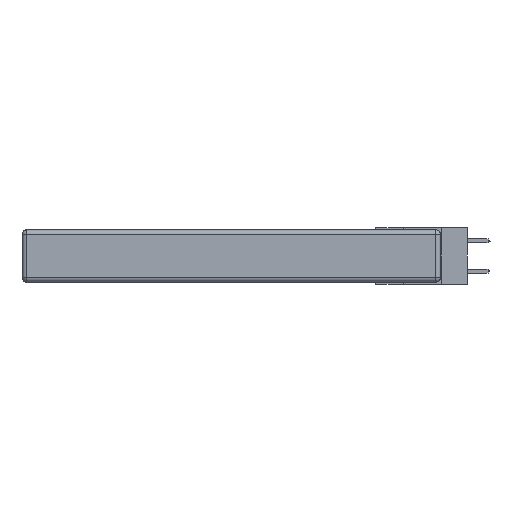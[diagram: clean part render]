
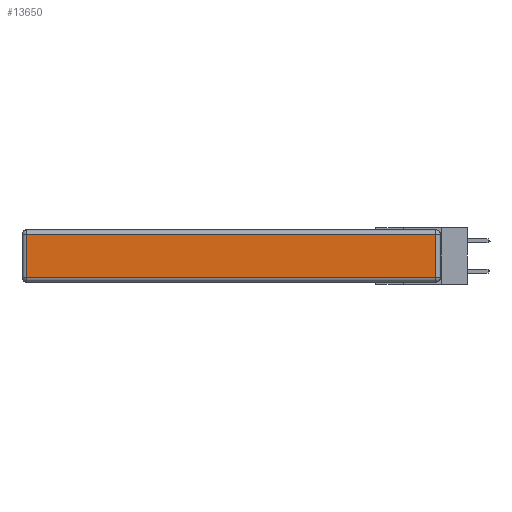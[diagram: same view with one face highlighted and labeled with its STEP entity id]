
A CAD part, left-side view. The second image highlights one B-rep face of the part: STEP entity #13650.
In plain terms, the highlighted planar face has unit normal (-1, 0, 0).
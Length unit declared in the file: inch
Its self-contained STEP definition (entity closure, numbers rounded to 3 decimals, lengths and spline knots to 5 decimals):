
#356 = CARTESIAN_POINT ( 'NONE',  ( 0., 2.75, -0.03 ) ) ;
#1478 = CARTESIAN_POINT ( 'NONE',  ( 0., 0.03, -0.343 ) ) ;
#2402 = VECTOR ( 'NONE', #15429, 39.37008 ) ;
#2646 = VECTOR ( 'NONE', #3074, 39.37008 ) ;
#2724 = EDGE_CURVE ( 'NONE', #3350, #12357, #8778, .T. ) ;
#3074 = DIRECTION ( 'NONE',  ( 0., -1., 0. ) ) ;
#3319 = LINE ( 'NONE', #356, #2402 ) ;
#3350 = VERTEX_POINT ( 'NONE', #22153 ) ;
#5187 = VECTOR ( 'NONE', #15113, 39.37008 ) ;
#5775 = FACE_OUTER_BOUND ( 'NONE', #20442, .T. ) ;
#5800 = LINE ( 'NONE', #1478, #5187 ) ;
#6814 = PLANE ( 'NONE',  #24048 ) ;
#8082 = LINE ( 'NONE', #13439, #24113 ) ;
#8778 = LINE ( 'NONE', #9116, #2646 ) ;
#9116 = CARTESIAN_POINT ( 'NONE',  ( 0., 0., -0.313 ) ) ;
#12357 = VERTEX_POINT ( 'NONE', #19832 ) ;
#13343 = EDGE_CURVE ( 'NONE', #12357, #22522, #5800, .T. ) ;
#13439 = CARTESIAN_POINT ( 'NONE',  ( 0., 2.72, -0.343 ) ) ;
#13650 = ADVANCED_FACE ( 'NONE', ( #5775 ), #6814, .T. ) ;
#13744 = CARTESIAN_POINT ( 'NONE',  ( 0., 2.72, -0.03 ) ) ;
#14708 = VERTEX_POINT ( 'NONE', #13744 ) ;
#15113 = DIRECTION ( 'NONE',  ( 0., 0., 1. ) ) ;
#15429 = DIRECTION ( 'NONE',  ( 0., 1., 0. ) ) ;
#16652 = DIRECTION ( 'NONE',  ( 0., 0., 1. ) ) ;
#17277 = EDGE_CURVE ( 'NONE', #14708, #3350, #8082, .T. ) ;
#17437 = DIRECTION ( 'NONE',  ( 0., 0., -1. ) ) ;
#18685 = DIRECTION ( 'NONE',  ( -1., 0., 0. ) ) ;
#19832 = CARTESIAN_POINT ( 'NONE',  ( 0., 0.03, -0.313 ) ) ;
#20442 = EDGE_LOOP ( 'NONE', ( #22126, #21494, #21517, #21757 ) ) ;
#21494 = ORIENTED_EDGE ( 'NONE', *, *, #13343, .T. ) ;
#21517 = ORIENTED_EDGE ( 'NONE', *, *, #23779, .T. ) ;
#21757 = ORIENTED_EDGE ( 'NONE', *, *, #17277, .T. ) ;
#22126 = ORIENTED_EDGE ( 'NONE', *, *, #2724, .T. ) ;
#22153 = CARTESIAN_POINT ( 'NONE',  ( 0., 2.72, -0.313 ) ) ;
#22172 = CARTESIAN_POINT ( 'NONE',  ( 0., 0., -0.343 ) ) ;
#22522 = VERTEX_POINT ( 'NONE', #23199 ) ;
#23199 = CARTESIAN_POINT ( 'NONE',  ( 0., 0.03, -0.03 ) ) ;
#23779 = EDGE_CURVE ( 'NONE', #22522, #14708, #3319, .T. ) ;
#24048 = AXIS2_PLACEMENT_3D ( 'NONE', #22172, #18685, #16652 ) ;
#24113 = VECTOR ( 'NONE', #17437, 39.37008 ) ;
